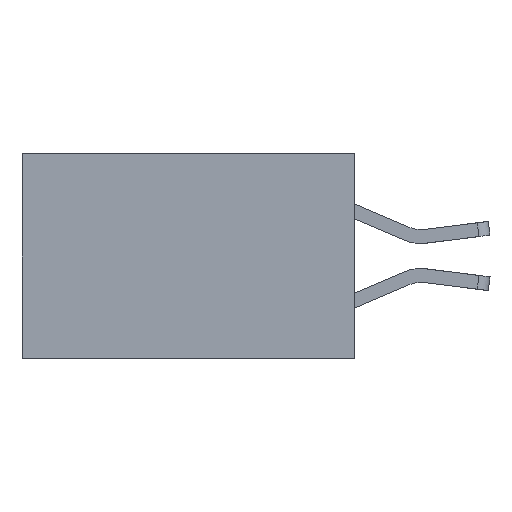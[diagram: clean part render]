
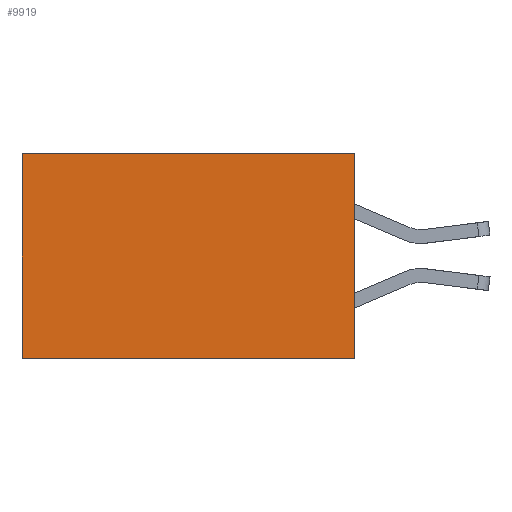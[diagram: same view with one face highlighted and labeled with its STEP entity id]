
A CAD part, left-side view. The second image highlights one B-rep face of the part: STEP entity #9919.
In plain terms, the highlighted planar face has unit normal (-1, 0, 0).
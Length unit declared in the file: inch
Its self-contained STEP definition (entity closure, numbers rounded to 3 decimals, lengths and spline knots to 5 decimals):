
#30 = CARTESIAN_POINT ( 'NONE',  ( 0.2615, 0., 0. ) ) ;
#376 = EDGE_CURVE ( 'NONE', #8881, #3966, #3307, .T. ) ;
#886 = VECTOR ( 'NONE', #3414, 39.37008 ) ;
#1206 = CARTESIAN_POINT ( 'NONE',  ( 0.2615, 0.6, 0. ) ) ;
#1381 = CARTESIAN_POINT ( 'NONE',  ( 0.2615, 0., -0.37 ) ) ;
#1585 = FACE_OUTER_BOUND ( 'NONE', #3941, .T. ) ;
#1634 = VERTEX_POINT ( 'NONE', #6046 ) ;
#2063 = CARTESIAN_POINT ( 'NONE',  ( 0.2615, 0., -0.37 ) ) ;
#2520 = CARTESIAN_POINT ( 'NONE',  ( 0.2615, 0., 0. ) ) ;
#2663 = EDGE_CURVE ( 'NONE', #6981, #1634, #9649, .T. ) ;
#2861 = VECTOR ( 'NONE', #3486, 39.37008 ) ;
#3147 = ORIENTED_EDGE ( 'NONE', *, *, #7449, .T. ) ;
#3307 = LINE ( 'NONE', #2520, #9794 ) ;
#3414 = DIRECTION ( 'NONE',  ( 0., 1., 0. ) ) ;
#3486 = DIRECTION ( 'NONE',  ( 0., 0., -1. ) ) ;
#3916 = DIRECTION ( 'NONE',  ( 0., 1., 0. ) ) ;
#3941 = EDGE_LOOP ( 'NONE', ( #3147, #5366, #7539, #9648 ) ) ;
#3966 = VERTEX_POINT ( 'NONE', #1206 ) ;
#3988 = DIRECTION ( 'NONE',  ( 1., 0., 0. ) ) ;
#4556 = CARTESIAN_POINT ( 'NONE',  ( 0.2615, 0., -0.37 ) ) ;
#4716 = DIRECTION ( 'NONE',  ( 0., 0., -1. ) ) ;
#4802 = AXIS2_PLACEMENT_3D ( 'NONE', #1381, #3988, #9641 ) ;
#5087 = LINE ( 'NONE', #5977, #2861 ) ;
#5366 = ORIENTED_EDGE ( 'NONE', *, *, #2663, .F. ) ;
#5447 = LINE ( 'NONE', #10316, #9719 ) ;
#5977 = CARTESIAN_POINT ( 'NONE',  ( 0.2615, 0.6, -0.37 ) ) ;
#6046 = CARTESIAN_POINT ( 'NONE',  ( 0.2615, 0.6, -0.37 ) ) ;
#6981 = VERTEX_POINT ( 'NONE', #2063 ) ;
#7449 = EDGE_CURVE ( 'NONE', #3966, #1634, #5087, .T. ) ;
#7539 = ORIENTED_EDGE ( 'NONE', *, *, #9259, .F. ) ;
#8837 = PLANE ( 'NONE',  #4802 ) ;
#8881 = VERTEX_POINT ( 'NONE', #30 ) ;
#9259 = EDGE_CURVE ( 'NONE', #8881, #6981, #5447, .T. ) ;
#9641 = DIRECTION ( 'NONE',  ( 0., 0., -1. ) ) ;
#9648 = ORIENTED_EDGE ( 'NONE', *, *, #376, .T. ) ;
#9649 = LINE ( 'NONE', #4556, #886 ) ;
#9719 = VECTOR ( 'NONE', #4716, 39.37008 ) ;
#9794 = VECTOR ( 'NONE', #3916, 39.37008 ) ;
#9919 = ADVANCED_FACE ( 'NONE', ( #1585 ), #8837, .F. ) ;
#10316 = CARTESIAN_POINT ( 'NONE',  ( 0.2615, 0., -0.37 ) ) ;
